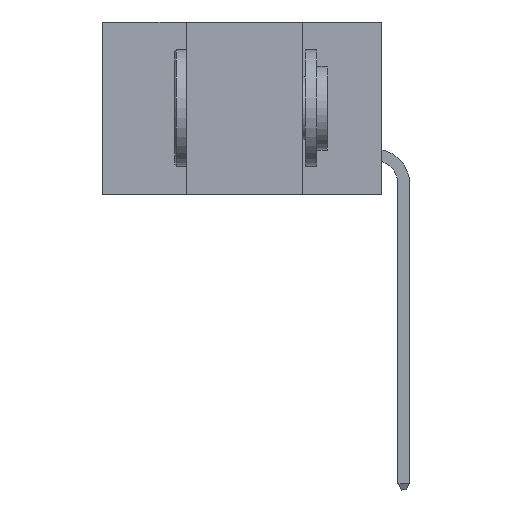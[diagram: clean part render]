
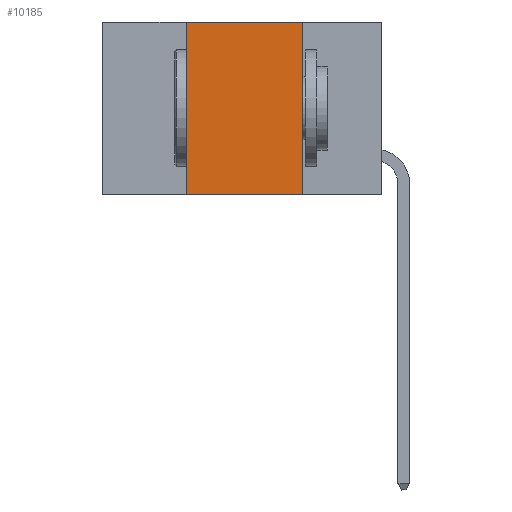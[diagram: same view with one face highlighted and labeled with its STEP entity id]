
A CAD part, left-side view. The second image highlights one B-rep face of the part: STEP entity #10185.
In plain terms, the highlighted planar face has unit normal (-1, 0, 0).
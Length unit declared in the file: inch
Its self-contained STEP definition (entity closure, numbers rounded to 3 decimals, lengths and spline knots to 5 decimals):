
#1067 = ORIENTED_EDGE ( 'NONE', *, *, #16854, .F. ) ;
#2260 = CARTESIAN_POINT ( 'NONE',  ( 0., 0.42, -0.37 ) ) ;
#3530 = FACE_OUTER_BOUND ( 'NONE', #23774, .T. ) ;
#3561 = EDGE_CURVE ( 'NONE', #25323, #3892, #18186, .T. ) ;
#3892 = VERTEX_POINT ( 'NONE', #8015 ) ;
#3920 = CARTESIAN_POINT ( 'NONE',  ( 0., 0.17, 0. ) ) ;
#4703 = ORIENTED_EDGE ( 'NONE', *, *, #16452, .F. ) ;
#7018 = CARTESIAN_POINT ( 'NONE',  ( 0., 0.6, 0. ) ) ;
#7095 = ORIENTED_EDGE ( 'NONE', *, *, #19793, .F. ) ;
#8015 = CARTESIAN_POINT ( 'NONE',  ( 0., 0.17, -0.37 ) ) ;
#8197 = VECTOR ( 'NONE', #23997, 39.37008 ) ;
#9370 = DIRECTION ( 'NONE',  ( 0., 0., 1. ) ) ;
#10185 = ADVANCED_FACE ( 'NONE', ( #3530 ), #16063, .F. ) ;
#10570 = VERTEX_POINT ( 'NONE', #13811 ) ;
#13811 = CARTESIAN_POINT ( 'NONE',  ( 0., 0.17, 0. ) ) ;
#14655 = VECTOR ( 'NONE', #22907, 39.37008 ) ;
#16063 = PLANE ( 'NONE',  #20248 ) ;
#16064 = VERTEX_POINT ( 'NONE', #23911 ) ;
#16447 = LINE ( 'NONE', #3920, #8197 ) ;
#16452 = EDGE_CURVE ( 'NONE', #25323, #16064, #24552, .T. ) ;
#16854 = EDGE_CURVE ( 'NONE', #16064, #10570, #25477, .T. ) ;
#18094 = DIRECTION ( 'NONE',  ( 1., 0., 0. ) ) ;
#18186 = LINE ( 'NONE', #24010, #22938 ) ;
#19404 = CARTESIAN_POINT ( 'NONE',  ( 0., 0.42, 0. ) ) ;
#19793 = EDGE_CURVE ( 'NONE', #10570, #3892, #16447, .T. ) ;
#20248 = AXIS2_PLACEMENT_3D ( 'NONE', #21841, #18094, #26066 ) ;
#20688 = ORIENTED_EDGE ( 'NONE', *, *, #3561, .T. ) ;
#21841 = CARTESIAN_POINT ( 'NONE',  ( 0., 0.6, 0. ) ) ;
#22907 = DIRECTION ( 'NONE',  ( 0., -1., 0. ) ) ;
#22938 = VECTOR ( 'NONE', #23756, 39.37008 ) ;
#22953 = VECTOR ( 'NONE', #9370, 39.37008 ) ;
#23756 = DIRECTION ( 'NONE',  ( 0., -1., 0. ) ) ;
#23774 = EDGE_LOOP ( 'NONE', ( #7095, #1067, #4703, #20688 ) ) ;
#23911 = CARTESIAN_POINT ( 'NONE',  ( 0., 0.42, 0. ) ) ;
#23997 = DIRECTION ( 'NONE',  ( 0., 0., -1. ) ) ;
#24010 = CARTESIAN_POINT ( 'NONE',  ( 0., 0.6, -0.37 ) ) ;
#24552 = LINE ( 'NONE', #19404, #22953 ) ;
#25323 = VERTEX_POINT ( 'NONE', #2260 ) ;
#25477 = LINE ( 'NONE', #7018, #14655 ) ;
#26066 = DIRECTION ( 'NONE',  ( 0., 0., -1. ) ) ;
